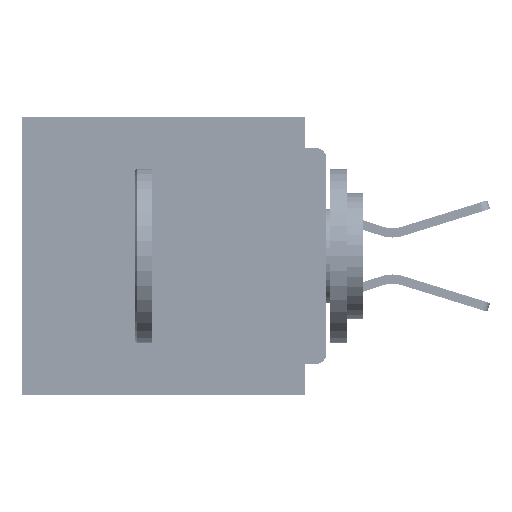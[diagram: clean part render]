
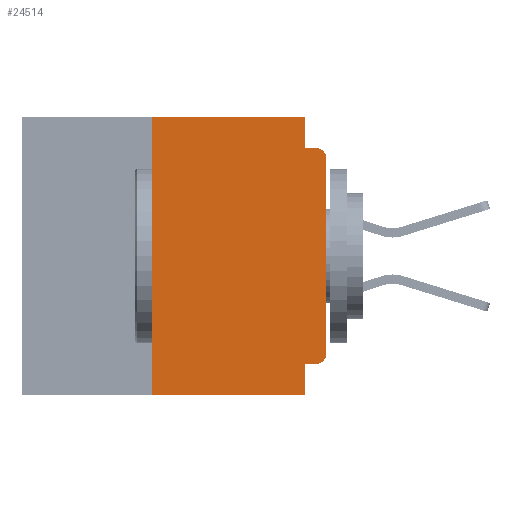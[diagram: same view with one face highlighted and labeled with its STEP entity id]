
A CAD part, left-side view. The second image highlights one B-rep face of the part: STEP entity #24514.
In plain terms, the highlighted planar face has unit normal (-1, 0, 0).
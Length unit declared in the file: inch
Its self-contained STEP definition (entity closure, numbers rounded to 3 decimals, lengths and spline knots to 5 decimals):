
#841 = VERTEX_POINT ( 'NONE', #63484 ) ;
#1004 = DIRECTION ( 'NONE',  ( 1., 0., 0. ) ) ;
#1077 = EDGE_CURVE ( 'NONE', #17764, #36345, #25943, .T. ) ;
#2140 = CARTESIAN_POINT ( 'NONE',  ( 0., 0.25, -0.4 ) ) ;
#2333 = EDGE_CURVE ( 'NONE', #17587, #37247, #65595, .T. ) ;
#2475 = CARTESIAN_POINT ( 'NONE',  ( 0., 0.437, 0. ) ) ;
#3556 = EDGE_CURVE ( 'NONE', #25738, #13495, #63063, .T. ) ;
#3620 = DIRECTION ( 'NONE',  ( 0., 0., 1. ) ) ;
#3809 = CARTESIAN_POINT ( 'NONE',  ( 0., 0.437, -0.4 ) ) ;
#8699 = EDGE_CURVE ( 'NONE', #34920, #33766, #50813, .T. ) ;
#10555 = EDGE_CURVE ( 'NONE', #841, #23644, #30671, .T. ) ;
#11162 = EDGE_LOOP ( 'NONE', ( #20450, #34355, #58300, #13132, #56627, #64726, #46085, #59562, #29015, #46842 ) ) ;
#11369 = LINE ( 'NONE', #2475, #50407 ) ;
#12383 = DIRECTION ( 'NONE',  ( -1., 0., 0. ) ) ;
#12882 = DIRECTION ( 'NONE',  ( 0., -1., 0. ) ) ;
#13132 = ORIENTED_EDGE ( 'NONE', *, *, #1077, .F. ) ;
#13495 = VERTEX_POINT ( 'NONE', #30959 ) ;
#14023 = CARTESIAN_POINT ( 'NONE',  ( 0., 0.015, -0.355 ) ) ;
#15397 = LINE ( 'NONE', #3809, #42479 ) ;
#16519 = EDGE_CURVE ( 'NONE', #34920, #841, #30686, .T. ) ;
#17147 = VECTOR ( 'NONE', #57747, 39.37008 ) ;
#17587 = VERTEX_POINT ( 'NONE', #64570 ) ;
#17764 = VERTEX_POINT ( 'NONE', #25312 ) ;
#20450 = ORIENTED_EDGE ( 'NONE', *, *, #34874, .T. ) ;
#20892 = CARTESIAN_POINT ( 'NONE',  ( 0., 0., -0.34 ) ) ;
#22042 = DIRECTION ( 'NONE',  ( 0., 1., 0. ) ) ;
#22184 = CARTESIAN_POINT ( 'NONE',  ( 0., 0.031, -0.4 ) ) ;
#23644 = VERTEX_POINT ( 'NONE', #40248 ) ;
#24014 = CARTESIAN_POINT ( 'NONE',  ( 0., 0., 0. ) ) ;
#24222 = VECTOR ( 'NONE', #47299, 39.37008 ) ;
#24514 = ADVANCED_FACE ( 'NONE', ( #37621 ), #46844, .F. ) ;
#25312 = CARTESIAN_POINT ( 'NONE',  ( 0., 0.031, 0. ) ) ;
#25738 = VERTEX_POINT ( 'NONE', #53089 ) ;
#25823 = LINE ( 'NONE', #42184, #24222 ) ;
#25943 = LINE ( 'NONE', #54260, #52967 ) ;
#26106 = CARTESIAN_POINT ( 'NONE',  ( 0., 0.031, -0.045 ) ) ;
#29015 = ORIENTED_EDGE ( 'NONE', *, *, #16519, .F. ) ;
#29156 = DIRECTION ( 'NONE',  ( 0., 0., 1. ) ) ;
#30671 = LINE ( 'NONE', #22184, #17147 ) ;
#30686 = LINE ( 'NONE', #57606, #44259 ) ;
#30959 = CARTESIAN_POINT ( 'NONE',  ( 0., 0.015, -0.045 ) ) ;
#31683 = CARTESIAN_POINT ( 'NONE',  ( 0., 0.437, 0. ) ) ;
#33766 = VERTEX_POINT ( 'NONE', #20892 ) ;
#34355 = ORIENTED_EDGE ( 'NONE', *, *, #3556, .T. ) ;
#34396 = LINE ( 'NONE', #24014, #59819 ) ;
#34874 = EDGE_CURVE ( 'NONE', #33766, #25738, #34396, .T. ) ;
#34920 = VERTEX_POINT ( 'NONE', #14023 ) ;
#36345 = VERTEX_POINT ( 'NONE', #26106 ) ;
#36820 = DIRECTION ( 'NONE',  ( 0., 0., -1. ) ) ;
#37247 = VERTEX_POINT ( 'NONE', #58624 ) ;
#37621 = FACE_OUTER_BOUND ( 'NONE', #11162, .T. ) ;
#38653 = VECTOR ( 'NONE', #3620, 39.37008 ) ;
#40248 = CARTESIAN_POINT ( 'NONE',  ( 0., 0.031, -0.4 ) ) ;
#40364 = AXIS2_PLACEMENT_3D ( 'NONE', #31683, #1004, #36820 ) ;
#42184 = CARTESIAN_POINT ( 'NONE',  ( 0., 0., -0.045 ) ) ;
#42310 = AXIS2_PLACEMENT_3D ( 'NONE', #51358, #51299, #51136 ) ;
#42479 = VECTOR ( 'NONE', #64821, 39.37008 ) ;
#42927 = CARTESIAN_POINT ( 'NONE',  ( 0., 0.015, -0.34 ) ) ;
#44259 = VECTOR ( 'NONE', #22042, 39.37008 ) ;
#46085 = ORIENTED_EDGE ( 'NONE', *, *, #48161, .T. ) ;
#46842 = ORIENTED_EDGE ( 'NONE', *, *, #8699, .T. ) ;
#46844 = PLANE ( 'NONE',  #40364 ) ;
#47299 = DIRECTION ( 'NONE',  ( 0., -1., 0. ) ) ;
#47958 = EDGE_CURVE ( 'NONE', #37247, #17764, #11369, .T. ) ;
#48016 = DIRECTION ( 'NONE',  ( 0., 0., -1. ) ) ;
#48161 = EDGE_CURVE ( 'NONE', #17587, #23644, #15397, .T. ) ;
#50352 = AXIS2_PLACEMENT_3D ( 'NONE', #42927, #12383, #48016 ) ;
#50407 = VECTOR ( 'NONE', #12882, 39.37008 ) ;
#50813 = CIRCLE ( 'NONE', #50352, 0.015 ) ;
#51136 = DIRECTION ( 'NONE',  ( 0., 0., -1. ) ) ;
#51299 = DIRECTION ( 'NONE',  ( -1., 0., 0. ) ) ;
#51358 = CARTESIAN_POINT ( 'NONE',  ( 0., 0.015, -0.06 ) ) ;
#52967 = VECTOR ( 'NONE', #54306, 39.37008 ) ;
#53089 = CARTESIAN_POINT ( 'NONE',  ( 0., 0., -0.06 ) ) ;
#54260 = CARTESIAN_POINT ( 'NONE',  ( 0., 0.031, 0. ) ) ;
#54306 = DIRECTION ( 'NONE',  ( 0., 0., -1. ) ) ;
#56559 = EDGE_CURVE ( 'NONE', #36345, #13495, #25823, .T. ) ;
#56627 = ORIENTED_EDGE ( 'NONE', *, *, #47958, .F. ) ;
#57606 = CARTESIAN_POINT ( 'NONE',  ( 0., 0., -0.355 ) ) ;
#57747 = DIRECTION ( 'NONE',  ( 0., 0., -1. ) ) ;
#58300 = ORIENTED_EDGE ( 'NONE', *, *, #56559, .F. ) ;
#58624 = CARTESIAN_POINT ( 'NONE',  ( 0., 0.25, 0. ) ) ;
#59562 = ORIENTED_EDGE ( 'NONE', *, *, #10555, .F. ) ;
#59819 = VECTOR ( 'NONE', #29156, 39.37008 ) ;
#63063 = CIRCLE ( 'NONE', #42310, 0.015 ) ;
#63484 = CARTESIAN_POINT ( 'NONE',  ( 0., 0.031, -0.355 ) ) ;
#64570 = CARTESIAN_POINT ( 'NONE',  ( 0., 0.25, -0.4 ) ) ;
#64726 = ORIENTED_EDGE ( 'NONE', *, *, #2333, .F. ) ;
#64821 = DIRECTION ( 'NONE',  ( 0., -1., 0. ) ) ;
#65595 = LINE ( 'NONE', #2140, #38653 ) ;
